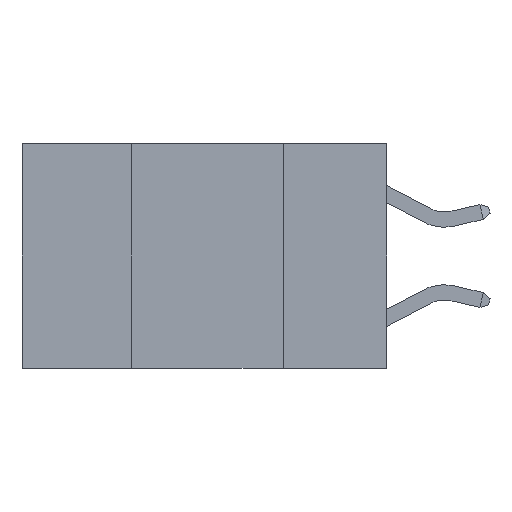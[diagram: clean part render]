
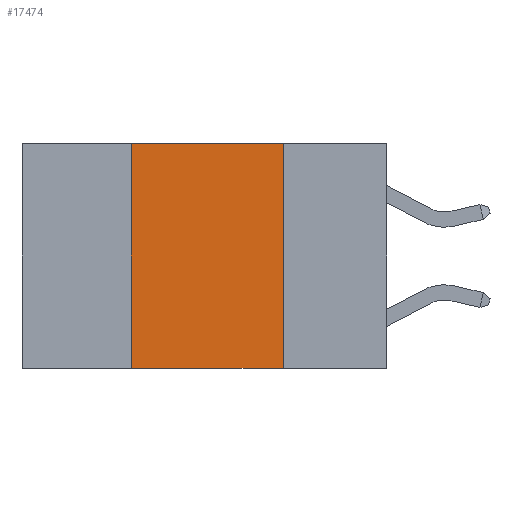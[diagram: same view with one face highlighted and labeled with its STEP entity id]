
A CAD part, left-side view. The second image highlights one B-rep face of the part: STEP entity #17474.
In plain terms, the highlighted planar face has unit normal (-1, 0, 0).
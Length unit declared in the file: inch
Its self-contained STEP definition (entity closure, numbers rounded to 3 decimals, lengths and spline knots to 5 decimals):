
#725 = VECTOR ( 'NONE', #20026, 39.37008 ) ;
#1624 = CARTESIAN_POINT ( 'NONE',  ( 0., 0.6, -0.37 ) ) ;
#2076 = EDGE_CURVE ( 'NONE', #13132, #15113, #5283, .T. ) ;
#2394 = VECTOR ( 'NONE', #4991, 39.37008 ) ;
#4464 = AXIS2_PLACEMENT_3D ( 'NONE', #19953, #12396, #17906 ) ;
#4991 = DIRECTION ( 'NONE',  ( 0., 0., 1. ) ) ;
#5283 = LINE ( 'NONE', #1624, #725 ) ;
#6085 = EDGE_CURVE ( 'NONE', #20179, #22452, #8125, .T. ) ;
#6305 = CARTESIAN_POINT ( 'NONE',  ( 0., 0.42, 0. ) ) ;
#8125 = LINE ( 'NONE', #15565, #21617 ) ;
#8692 = ORIENTED_EDGE ( 'NONE', *, *, #6085, .F. ) ;
#9392 = CARTESIAN_POINT ( 'NONE',  ( 0., 0.17, 0. ) ) ;
#9737 = EDGE_LOOP ( 'NONE', ( #17195, #8692, #11805, #22928 ) ) ;
#10166 = DIRECTION ( 'NONE',  ( 0., 0., -1. ) ) ;
#11373 = VECTOR ( 'NONE', #10166, 39.37008 ) ;
#11805 = ORIENTED_EDGE ( 'NONE', *, *, #14552, .F. ) ;
#11871 = CARTESIAN_POINT ( 'NONE',  ( 0., 0.17, 0. ) ) ;
#12396 = DIRECTION ( 'NONE',  ( 1., 0., 0. ) ) ;
#13132 = VERTEX_POINT ( 'NONE', #13535 ) ;
#13535 = CARTESIAN_POINT ( 'NONE',  ( 0., 0.42, -0.37 ) ) ;
#14552 = EDGE_CURVE ( 'NONE', #13132, #20179, #17928, .T. ) ;
#14884 = EDGE_CURVE ( 'NONE', #22452, #15113, #21152, .T. ) ;
#15113 = VERTEX_POINT ( 'NONE', #16767 ) ;
#15565 = CARTESIAN_POINT ( 'NONE',  ( 0., 0.6, 0. ) ) ;
#16068 = PLANE ( 'NONE',  #4464 ) ;
#16767 = CARTESIAN_POINT ( 'NONE',  ( 0., 0.17, -0.37 ) ) ;
#17195 = ORIENTED_EDGE ( 'NONE', *, *, #14884, .F. ) ;
#17474 = ADVANCED_FACE ( 'NONE', ( #21550 ), #16068, .F. ) ;
#17906 = DIRECTION ( 'NONE',  ( 0., 0., -1. ) ) ;
#17928 = LINE ( 'NONE', #21696, #2394 ) ;
#19953 = CARTESIAN_POINT ( 'NONE',  ( 0., 0.6, 0. ) ) ;
#20026 = DIRECTION ( 'NONE',  ( 0., -1., 0. ) ) ;
#20179 = VERTEX_POINT ( 'NONE', #6305 ) ;
#21152 = LINE ( 'NONE', #11871, #11373 ) ;
#21550 = FACE_OUTER_BOUND ( 'NONE', #9737, .T. ) ;
#21617 = VECTOR ( 'NONE', #23007, 39.37008 ) ;
#21696 = CARTESIAN_POINT ( 'NONE',  ( 0., 0.42, 0. ) ) ;
#22452 = VERTEX_POINT ( 'NONE', #9392 ) ;
#22928 = ORIENTED_EDGE ( 'NONE', *, *, #2076, .T. ) ;
#23007 = DIRECTION ( 'NONE',  ( 0., -1., 0. ) ) ;
